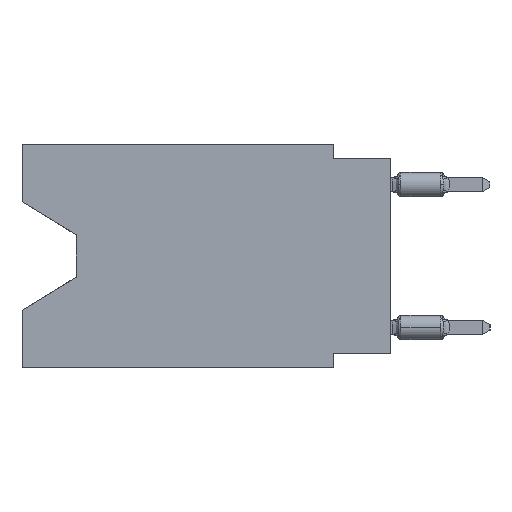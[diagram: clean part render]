
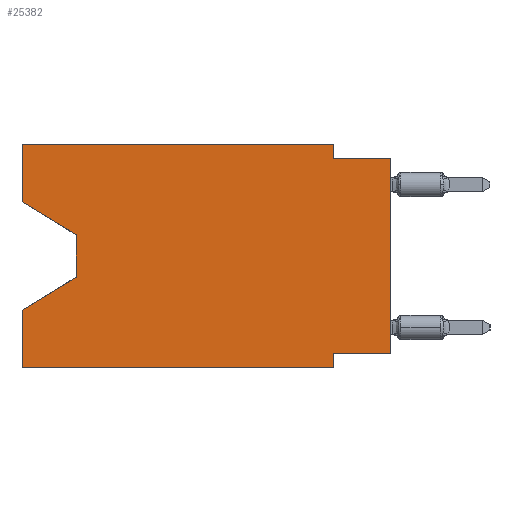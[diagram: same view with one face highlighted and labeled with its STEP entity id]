
A CAD part, left-side view. The second image highlights one B-rep face of the part: STEP entity #25382.
In plain terms, the highlighted planar face has unit normal (-1, 0, 0).
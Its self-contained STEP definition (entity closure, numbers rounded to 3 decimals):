
#859 = DIRECTION ( 'NONE',  ( 0., -0.855, -0.519 ) ) ;
#1042 = DIRECTION ( 'NONE',  ( 0., 0., -1. ) ) ;
#1629 = CARTESIAN_POINT ( 'NONE',  ( 0., 13.97, -5.893 ) ) ;
#1709 = LINE ( 'NONE', #4511, #34931 ) ;
#1720 = CARTESIAN_POINT ( 'NONE',  ( 0., 2.54, -9.906 ) ) ;
#1754 = ORIENTED_EDGE ( 'NONE', *, *, #4510, .F. ) ;
#2977 = DIRECTION ( 'NONE',  ( 1., 0., 0. ) ) ;
#3401 = CARTESIAN_POINT ( 'NONE',  ( 0., 16.383, 0. ) ) ;
#3694 = EDGE_LOOP ( 'NONE', ( #18681, #14597, #19832, #33140, #15048, #1754, #21849, #9375, #28449, #4497, #33696, #19981 ) ) ;
#3823 = CARTESIAN_POINT ( 'NONE',  ( 0., 0., -9.271 ) ) ;
#4497 = ORIENTED_EDGE ( 'NONE', *, *, #24178, .F. ) ;
#4510 = EDGE_CURVE ( 'NONE', #17748, #19030, #24643, .T. ) ;
#4511 = CARTESIAN_POINT ( 'NONE',  ( 0., 0., -9.271 ) ) ;
#4765 = EDGE_CURVE ( 'NONE', #13467, #19030, #29965, .T. ) ;
#4901 = DIRECTION ( 'NONE',  ( 0., -1., 0. ) ) ;
#6250 = CARTESIAN_POINT ( 'NONE',  ( 0., 16.383, -9.906 ) ) ;
#6378 = VECTOR ( 'NONE', #37285, 1000. ) ;
#6676 = LINE ( 'NONE', #15914, #8769 ) ;
#7284 = DIRECTION ( 'NONE',  ( 0., 0., 1. ) ) ;
#7731 = EDGE_CURVE ( 'NONE', #35827, #36965, #40095, .T. ) ;
#7935 = VERTEX_POINT ( 'NONE', #29113 ) ;
#8101 = DIRECTION ( 'NONE',  ( 0., 0.855, -0.519 ) ) ;
#8769 = VECTOR ( 'NONE', #38860, 1000. ) ;
#9375 = ORIENTED_EDGE ( 'NONE', *, *, #41986, .T. ) ;
#10524 = LINE ( 'NONE', #36695, #11661 ) ;
#10665 = VERTEX_POINT ( 'NONE', #23234 ) ;
#10740 = CARTESIAN_POINT ( 'NONE',  ( 0., 16.383, -2.546 ) ) ;
#11661 = VECTOR ( 'NONE', #7284, 1000. ) ;
#12338 = LINE ( 'NONE', #31458, #20036 ) ;
#12645 = FACE_OUTER_BOUND ( 'NONE', #3694, .T. ) ;
#12877 = EDGE_CURVE ( 'NONE', #16358, #35827, #12338, .T. ) ;
#13452 = EDGE_CURVE ( 'NONE', #13467, #10665, #6676, .T. ) ;
#13467 = VERTEX_POINT ( 'NONE', #6250 ) ;
#13819 = CARTESIAN_POINT ( 'NONE',  ( 0., 13.97, -4.013 ) ) ;
#14597 = ORIENTED_EDGE ( 'NONE', *, *, #40245, .T. ) ;
#15048 = ORIENTED_EDGE ( 'NONE', *, *, #4765, .T. ) ;
#15914 = CARTESIAN_POINT ( 'NONE',  ( 0., 16.383, 0. ) ) ;
#16358 = VERTEX_POINT ( 'NONE', #25508 ) ;
#17035 = LINE ( 'NONE', #13819, #26006 ) ;
#17748 = VERTEX_POINT ( 'NONE', #25516 ) ;
#18681 = ORIENTED_EDGE ( 'NONE', *, *, #36277, .T. ) ;
#18855 = CARTESIAN_POINT ( 'NONE',  ( 0., 2.54, 0. ) ) ;
#19030 = VERTEX_POINT ( 'NONE', #1720 ) ;
#19832 = ORIENTED_EDGE ( 'NONE', *, *, #22585, .T. ) ;
#19981 = ORIENTED_EDGE ( 'NONE', *, *, #12877, .F. ) ;
#20036 = VECTOR ( 'NONE', #41314, 1000. ) ;
#20048 = VERTEX_POINT ( 'NONE', #1629 ) ;
#20644 = VERTEX_POINT ( 'NONE', #3823 ) ;
#21240 = CARTESIAN_POINT ( 'NONE',  ( 0., 2.54, -0.635 ) ) ;
#21390 = VECTOR ( 'NONE', #1042, 1000. ) ;
#21849 = ORIENTED_EDGE ( 'NONE', *, *, #42144, .F. ) ;
#22585 = EDGE_CURVE ( 'NONE', #20048, #10665, #33642, .T. ) ;
#22926 = PLANE ( 'NONE',  #37862 ) ;
#23234 = CARTESIAN_POINT ( 'NONE',  ( 0., 16.383, -7.36 ) ) ;
#23687 = DIRECTION ( 'NONE',  ( 0., 0., -1. ) ) ;
#23879 = VECTOR ( 'NONE', #4901, 1000. ) ;
#23989 = DIRECTION ( 'NONE',  ( 0., 0., -1. ) ) ;
#24178 = EDGE_CURVE ( 'NONE', #36965, #25220, #38591, .T. ) ;
#24195 = CARTESIAN_POINT ( 'NONE',  ( 0., 0., -0.635 ) ) ;
#24643 = LINE ( 'NONE', #30459, #21390 ) ;
#25220 = VERTEX_POINT ( 'NONE', #21240 ) ;
#25382 = ADVANCED_FACE ( 'NONE', ( #12645 ), #22926, .F. ) ;
#25508 = CARTESIAN_POINT ( 'NONE',  ( 0., 16.383, -2.546 ) ) ;
#25516 = CARTESIAN_POINT ( 'NONE',  ( 0., 2.54, -9.271 ) ) ;
#26006 = VECTOR ( 'NONE', #23687, 1000. ) ;
#26098 = VECTOR ( 'NONE', #23989, 1000. ) ;
#27306 = CARTESIAN_POINT ( 'NONE',  ( 0., 16.383, 0. ) ) ;
#28449 = ORIENTED_EDGE ( 'NONE', *, *, #33858, .F. ) ;
#28483 = VECTOR ( 'NONE', #859, 1000. ) ;
#29113 = CARTESIAN_POINT ( 'NONE',  ( 0., 0., -0.635 ) ) ;
#29965 = LINE ( 'NONE', #36196, #33102 ) ;
#30432 = CARTESIAN_POINT ( 'NONE',  ( 0., 13.97, -5.893 ) ) ;
#30459 = CARTESIAN_POINT ( 'NONE',  ( 0., 2.54, -9.906 ) ) ;
#31458 = CARTESIAN_POINT ( 'NONE',  ( 0., 16.383, 0. ) ) ;
#31888 = CARTESIAN_POINT ( 'NONE',  ( 0., 13.97, -4.013 ) ) ;
#32169 = DIRECTION ( 'NONE',  ( 0., 0., -1. ) ) ;
#32311 = VECTOR ( 'NONE', #8101, 1000. ) ;
#32691 = CARTESIAN_POINT ( 'NONE',  ( 0., 2.54, 0. ) ) ;
#33102 = VECTOR ( 'NONE', #39621, 1000. ) ;
#33140 = ORIENTED_EDGE ( 'NONE', *, *, #13452, .F. ) ;
#33635 = LINE ( 'NONE', #24195, #6378 ) ;
#33642 = LINE ( 'NONE', #30432, #32311 ) ;
#33696 = ORIENTED_EDGE ( 'NONE', *, *, #7731, .F. ) ;
#33858 = EDGE_CURVE ( 'NONE', #25220, #7935, #33635, .T. ) ;
#34931 = VECTOR ( 'NONE', #40338, 1000. ) ;
#35827 = VERTEX_POINT ( 'NONE', #27306 ) ;
#36196 = CARTESIAN_POINT ( 'NONE',  ( 0., 16.383, -9.906 ) ) ;
#36277 = EDGE_CURVE ( 'NONE', #16358, #41186, #36703, .T. ) ;
#36668 = CARTESIAN_POINT ( 'NONE',  ( 0., 16.383, 0. ) ) ;
#36695 = CARTESIAN_POINT ( 'NONE',  ( 0., 0., 0. ) ) ;
#36703 = LINE ( 'NONE', #10740, #28483 ) ;
#36965 = VERTEX_POINT ( 'NONE', #32691 ) ;
#37285 = DIRECTION ( 'NONE',  ( 0., -1., 0. ) ) ;
#37862 = AXIS2_PLACEMENT_3D ( 'NONE', #3401, #2977, #32169 ) ;
#38591 = LINE ( 'NONE', #18855, #26098 ) ;
#38860 = DIRECTION ( 'NONE',  ( 0., 0., 1. ) ) ;
#39621 = DIRECTION ( 'NONE',  ( 0., -1., 0. ) ) ;
#40095 = LINE ( 'NONE', #36668, #23879 ) ;
#40245 = EDGE_CURVE ( 'NONE', #41186, #20048, #17035, .T. ) ;
#40338 = DIRECTION ( 'NONE',  ( 0., 1., 0. ) ) ;
#41186 = VERTEX_POINT ( 'NONE', #31888 ) ;
#41314 = DIRECTION ( 'NONE',  ( 0., 0., 1. ) ) ;
#41986 = EDGE_CURVE ( 'NONE', #20644, #7935, #10524, .T. ) ;
#42144 = EDGE_CURVE ( 'NONE', #20644, #17748, #1709, .T. ) ;
